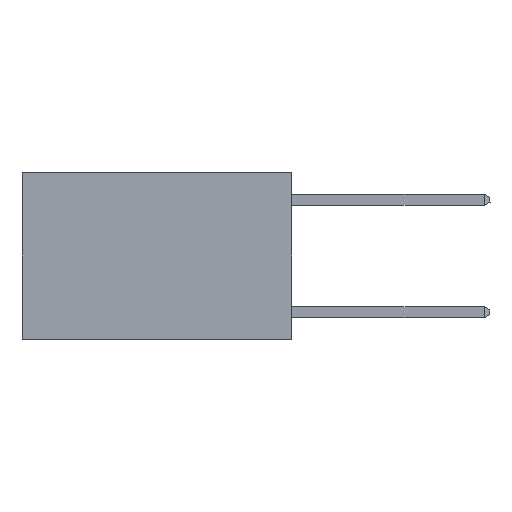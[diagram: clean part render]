
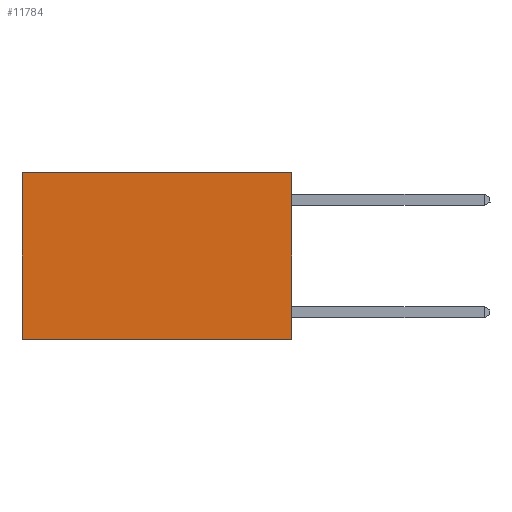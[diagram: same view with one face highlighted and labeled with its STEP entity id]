
A CAD part, left-side view. The second image highlights one B-rep face of the part: STEP entity #11784.
In plain terms, the highlighted planar face has unit normal (-1, 0, 0).
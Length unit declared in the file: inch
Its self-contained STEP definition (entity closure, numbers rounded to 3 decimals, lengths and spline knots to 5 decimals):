
#326 = CARTESIAN_POINT ( 'NONE',  ( 0.2625, 0.6, 0. ) ) ;
#356 = CARTESIAN_POINT ( 'NONE',  ( 0.2625, 0.6, 0. ) ) ;
#544 = FACE_OUTER_BOUND ( 'NONE', #7073, .T. ) ;
#2510 = ORIENTED_EDGE ( 'NONE', *, *, #5277, .T. ) ;
#2741 = LINE ( 'NONE', #326, #13347 ) ;
#4157 = VECTOR ( 'NONE', #9280, 39.37008 ) ;
#4311 = VERTEX_POINT ( 'NONE', #356 ) ;
#4353 = DIRECTION ( 'NONE',  ( 1., 0., 0. ) ) ;
#4591 = LINE ( 'NONE', #8151, #15203 ) ;
#4823 = DIRECTION ( 'NONE',  ( 0., 0., -1. ) ) ;
#5249 = ORIENTED_EDGE ( 'NONE', *, *, #8603, .F. ) ;
#5277 = EDGE_CURVE ( 'NONE', #14189, #4311, #4591, .T. ) ;
#5291 = VERTEX_POINT ( 'NONE', #5761 ) ;
#5484 = LINE ( 'NONE', #15537, #4157 ) ;
#5761 = CARTESIAN_POINT ( 'NONE',  ( 0.2625, 0., -0.37 ) ) ;
#5866 = ORIENTED_EDGE ( 'NONE', *, *, #12673, .F. ) ;
#7068 = DIRECTION ( 'NONE',  ( 0., 1., 0. ) ) ;
#7073 = EDGE_LOOP ( 'NONE', ( #13726, #5866, #5249, #2510 ) ) ;
#7287 = CARTESIAN_POINT ( 'NONE',  ( 0.2625, 0., 0. ) ) ;
#8151 = CARTESIAN_POINT ( 'NONE',  ( 0.2625, 0., 0. ) ) ;
#8603 = EDGE_CURVE ( 'NONE', #14189, #5291, #9772, .T. ) ;
#9280 = DIRECTION ( 'NONE',  ( 0., 1., 0. ) ) ;
#9772 = LINE ( 'NONE', #7287, #10229 ) ;
#10229 = VECTOR ( 'NONE', #4823, 39.37008 ) ;
#10585 = EDGE_CURVE ( 'NONE', #4311, #11786, #2741, .T. ) ;
#10635 = PLANE ( 'NONE',  #15841 ) ;
#11665 = DIRECTION ( 'NONE',  ( 0., 0., -1. ) ) ;
#11784 = ADVANCED_FACE ( 'NONE', ( #544 ), #10635, .F. ) ;
#11786 = VERTEX_POINT ( 'NONE', #14440 ) ;
#12563 = CARTESIAN_POINT ( 'NONE',  ( 0.2625, 0., 0. ) ) ;
#12673 = EDGE_CURVE ( 'NONE', #5291, #11786, #5484, .T. ) ;
#13279 = CARTESIAN_POINT ( 'NONE',  ( 0.2625, 0., 0. ) ) ;
#13347 = VECTOR ( 'NONE', #11665, 39.37008 ) ;
#13726 = ORIENTED_EDGE ( 'NONE', *, *, #10585, .T. ) ;
#14189 = VERTEX_POINT ( 'NONE', #12563 ) ;
#14440 = CARTESIAN_POINT ( 'NONE',  ( 0.2625, 0.6, -0.37 ) ) ;
#15203 = VECTOR ( 'NONE', #7068, 39.37008 ) ;
#15537 = CARTESIAN_POINT ( 'NONE',  ( 0.2625, 0., -0.37 ) ) ;
#15657 = DIRECTION ( 'NONE',  ( 0., 0., -1. ) ) ;
#15841 = AXIS2_PLACEMENT_3D ( 'NONE', #13279, #4353, #15657 ) ;
